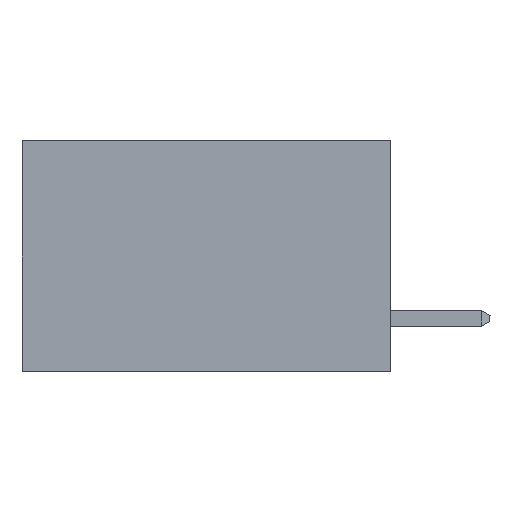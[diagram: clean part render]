
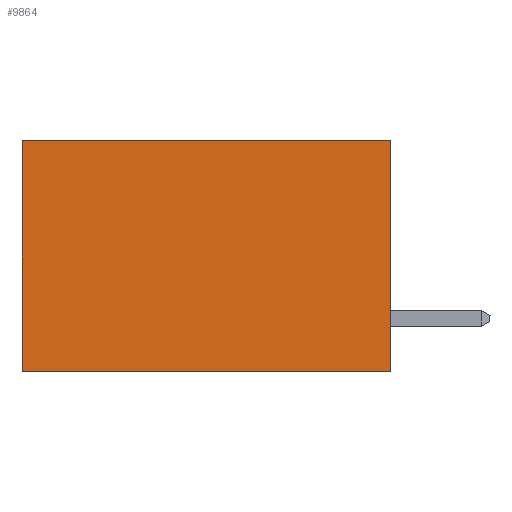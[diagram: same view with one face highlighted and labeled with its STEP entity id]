
A CAD part, left-side view. The second image highlights one B-rep face of the part: STEP entity #9864.
In plain terms, the highlighted planar face has unit normal (-1, 0, 0).
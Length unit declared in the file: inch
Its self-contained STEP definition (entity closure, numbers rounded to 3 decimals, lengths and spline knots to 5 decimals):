
#633 = DIRECTION ( 'NONE',  ( 1., 0., 0. ) ) ;
#1026 = VERTEX_POINT ( 'NONE', #2031 ) ;
#1300 = ORIENTED_EDGE ( 'NONE', *, *, #6601, .F. ) ;
#2031 = CARTESIAN_POINT ( 'NONE',  ( 0.277, 0.59, -0.37 ) ) ;
#2275 = PLANE ( 'NONE',  #10453 ) ;
#2322 = LINE ( 'NONE', #5188, #4581 ) ;
#2733 = LINE ( 'NONE', #8108, #9097 ) ;
#2787 = CARTESIAN_POINT ( 'NONE',  ( 0.277, 0., 0. ) ) ;
#2810 = VERTEX_POINT ( 'NONE', #2787 ) ;
#2876 = CARTESIAN_POINT ( 'NONE',  ( 0.277, 0., -0.37 ) ) ;
#3482 = CARTESIAN_POINT ( 'NONE',  ( 0.277, 0., 0. ) ) ;
#3499 = ORIENTED_EDGE ( 'NONE', *, *, #9678, .F. ) ;
#3613 = DIRECTION ( 'NONE',  ( 0., 1., 0. ) ) ;
#3737 = DIRECTION ( 'NONE',  ( 0., 1., 0. ) ) ;
#4581 = VECTOR ( 'NONE', #5156, 39.37008 ) ;
#4582 = VECTOR ( 'NONE', #3613, 39.37008 ) ;
#5117 = LINE ( 'NONE', #2876, #8707 ) ;
#5156 = DIRECTION ( 'NONE',  ( 0., 0., -1. ) ) ;
#5188 = CARTESIAN_POINT ( 'NONE',  ( 0.277, 0.59, -0.37 ) ) ;
#5554 = EDGE_LOOP ( 'NONE', ( #7412, #3499, #1300, #10706 ) ) ;
#5673 = CARTESIAN_POINT ( 'NONE',  ( 0.277, 0., -0.37 ) ) ;
#5801 = VERTEX_POINT ( 'NONE', #8678 ) ;
#6502 = DIRECTION ( 'NONE',  ( 0., 0., -1. ) ) ;
#6601 = EDGE_CURVE ( 'NONE', #2810, #5801, #2733, .T. ) ;
#6900 = EDGE_CURVE ( 'NONE', #10573, #1026, #2322, .T. ) ;
#7093 = FACE_OUTER_BOUND ( 'NONE', #5554, .T. ) ;
#7412 = ORIENTED_EDGE ( 'NONE', *, *, #6900, .T. ) ;
#7524 = EDGE_CURVE ( 'NONE', #2810, #10573, #8971, .T. ) ;
#8108 = CARTESIAN_POINT ( 'NONE',  ( 0.277, 0., -0.37 ) ) ;
#8344 = DIRECTION ( 'NONE',  ( 0., 0., -1. ) ) ;
#8678 = CARTESIAN_POINT ( 'NONE',  ( 0.277, 0., -0.37 ) ) ;
#8707 = VECTOR ( 'NONE', #3737, 39.37008 ) ;
#8971 = LINE ( 'NONE', #3482, #4582 ) ;
#9030 = CARTESIAN_POINT ( 'NONE',  ( 0.277, 0.59, 0. ) ) ;
#9097 = VECTOR ( 'NONE', #8344, 39.37008 ) ;
#9678 = EDGE_CURVE ( 'NONE', #5801, #1026, #5117, .T. ) ;
#9864 = ADVANCED_FACE ( 'NONE', ( #7093 ), #2275, .F. ) ;
#10453 = AXIS2_PLACEMENT_3D ( 'NONE', #5673, #633, #6502 ) ;
#10573 = VERTEX_POINT ( 'NONE', #9030 ) ;
#10706 = ORIENTED_EDGE ( 'NONE', *, *, #7524, .T. ) ;
